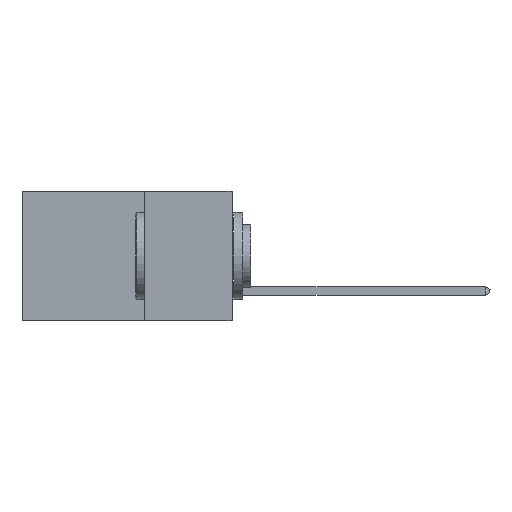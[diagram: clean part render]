
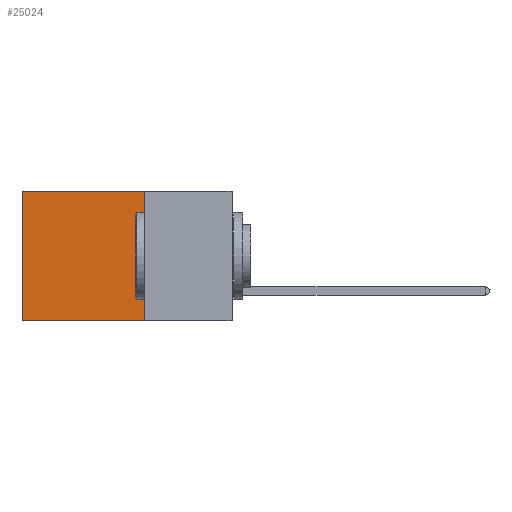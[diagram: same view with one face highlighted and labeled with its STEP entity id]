
A CAD part, left-side view. The second image highlights one B-rep face of the part: STEP entity #25024.
In plain terms, the highlighted planar face has unit normal (-1, 0, 0).
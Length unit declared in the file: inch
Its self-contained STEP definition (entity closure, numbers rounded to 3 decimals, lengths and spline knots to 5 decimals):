
#1213 = AXIS2_PLACEMENT_3D ( 'NONE', #27305, #23181, #32986 ) ;
#2287 = VERTEX_POINT ( 'NONE', #14578 ) ;
#2323 = VERTEX_POINT ( 'NONE', #23991 ) ;
#2365 = ORIENTED_EDGE ( 'NONE', *, *, #18053, .F. ) ;
#3070 = LINE ( 'NONE', #23780, #7220 ) ;
#3524 = FACE_OUTER_BOUND ( 'NONE', #16218, .T. ) ;
#3536 = ORIENTED_EDGE ( 'NONE', *, *, #16523, .T. ) ;
#3549 = PLANE ( 'NONE',  #1213 ) ;
#5113 = ORIENTED_EDGE ( 'NONE', *, *, #33478, .T. ) ;
#5990 = VERTEX_POINT ( 'NONE', #31480 ) ;
#7220 = VECTOR ( 'NONE', #31460, 39.37008 ) ;
#7422 = CARTESIAN_POINT ( 'NONE',  ( 0.2875, 0.25, 0. ) ) ;
#8936 = LINE ( 'NONE', #7422, #15138 ) ;
#14463 = EDGE_CURVE ( 'NONE', #5990, #23907, #33851, .T. ) ;
#14533 = ORIENTED_EDGE ( 'NONE', *, *, #14463, .F. ) ;
#14578 = CARTESIAN_POINT ( 'NONE',  ( 0.2875, 0.6, -0.37 ) ) ;
#15138 = VECTOR ( 'NONE', #18169, 39.37008 ) ;
#15364 = DIRECTION ( 'NONE',  ( 0., 0., -1. ) ) ;
#16218 = EDGE_LOOP ( 'NONE', ( #5113, #2365, #14533, #3536 ) ) ;
#16523 = EDGE_CURVE ( 'NONE', #5990, #2323, #8936, .T. ) ;
#17814 = VECTOR ( 'NONE', #32075, 39.37008 ) ;
#18053 = EDGE_CURVE ( 'NONE', #23907, #2287, #3070, .T. ) ;
#18169 = DIRECTION ( 'NONE',  ( 0., 1., 0. ) ) ;
#18988 = VECTOR ( 'NONE', #15364, 39.37008 ) ;
#20471 = CARTESIAN_POINT ( 'NONE',  ( 0.2875, 0.25, 0. ) ) ;
#20690 = LINE ( 'NONE', #24143, #17814 ) ;
#22931 = CARTESIAN_POINT ( 'NONE',  ( 0.2875, 0.25, -0.37 ) ) ;
#23181 = DIRECTION ( 'NONE',  ( 1., 0., 0. ) ) ;
#23780 = CARTESIAN_POINT ( 'NONE',  ( 0.2875, 0.25, -0.37 ) ) ;
#23907 = VERTEX_POINT ( 'NONE', #22931 ) ;
#23991 = CARTESIAN_POINT ( 'NONE',  ( 0.2875, 0.6, 0. ) ) ;
#24143 = CARTESIAN_POINT ( 'NONE',  ( 0.2875, 0.6, 0. ) ) ;
#25024 = ADVANCED_FACE ( 'NONE', ( #3524 ), #3549, .F. ) ;
#27305 = CARTESIAN_POINT ( 'NONE',  ( 0.2875, 0.25, 0. ) ) ;
#31460 = DIRECTION ( 'NONE',  ( 0., 1., 0. ) ) ;
#31480 = CARTESIAN_POINT ( 'NONE',  ( 0.2875, 0.25, 0. ) ) ;
#32075 = DIRECTION ( 'NONE',  ( 0., 0., -1. ) ) ;
#32986 = DIRECTION ( 'NONE',  ( 0., 0., -1. ) ) ;
#33478 = EDGE_CURVE ( 'NONE', #2323, #2287, #20690, .T. ) ;
#33851 = LINE ( 'NONE', #20471, #18988 ) ;
